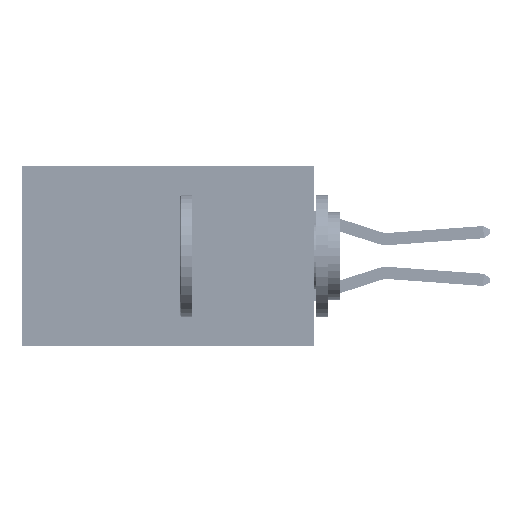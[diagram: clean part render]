
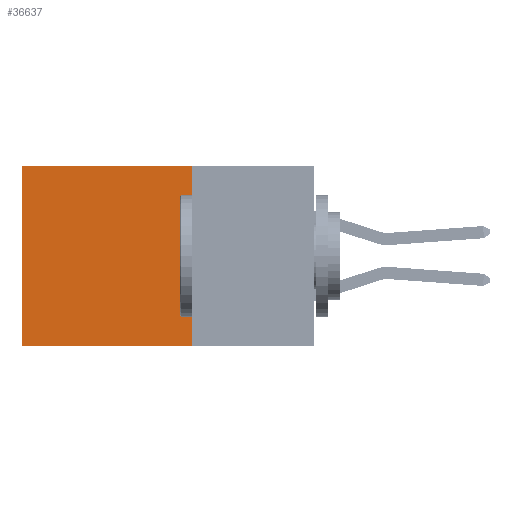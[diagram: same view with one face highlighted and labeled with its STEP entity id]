
A CAD part, left-side view. The second image highlights one B-rep face of the part: STEP entity #36637.
In plain terms, the highlighted planar face has unit normal (-1, 0, 0).
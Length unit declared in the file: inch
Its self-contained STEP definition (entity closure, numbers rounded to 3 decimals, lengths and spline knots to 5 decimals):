
#1279 = CARTESIAN_POINT ( 'NONE',  ( 0.2875, 0.25, 0. ) ) ;
#1438 = DIRECTION ( 'NONE',  ( 0., 1., 0. ) ) ;
#1686 = CARTESIAN_POINT ( 'NONE',  ( 0.2875, 0.6, 0. ) ) ;
#4145 = VERTEX_POINT ( 'NONE', #43274 ) ;
#5166 = DIRECTION ( 'NONE',  ( 1., 0., 0. ) ) ;
#6476 = CARTESIAN_POINT ( 'NONE',  ( 0.2875, 0.25, 0. ) ) ;
#7086 = LINE ( 'NONE', #35724, #45134 ) ;
#7599 = LINE ( 'NONE', #1686, #35656 ) ;
#8905 = ORIENTED_EDGE ( 'NONE', *, *, #9868, .T. ) ;
#8907 = PLANE ( 'NONE',  #10099 ) ;
#9868 = EDGE_CURVE ( 'NONE', #30553, #10388, #7599, .T. ) ;
#10099 = AXIS2_PLACEMENT_3D ( 'NONE', #1279, #5166, #31964 ) ;
#10341 = ORIENTED_EDGE ( 'NONE', *, *, #35509, .F. ) ;
#10388 = VERTEX_POINT ( 'NONE', #43488 ) ;
#11145 = VERTEX_POINT ( 'NONE', #36205 ) ;
#11567 = DIRECTION ( 'NONE',  ( 0., 1., 0. ) ) ;
#13233 = VECTOR ( 'NONE', #21738, 39.37008 ) ;
#17174 = DIRECTION ( 'NONE',  ( 0., 0., -1. ) ) ;
#19531 = ORIENTED_EDGE ( 'NONE', *, *, #38945, .T. ) ;
#21738 = DIRECTION ( 'NONE',  ( 0., 0., -1. ) ) ;
#23181 = VECTOR ( 'NONE', #11567, 39.37008 ) ;
#25744 = EDGE_LOOP ( 'NONE', ( #8905, #36055, #10341, #19531 ) ) ;
#30553 = VERTEX_POINT ( 'NONE', #30928 ) ;
#30922 = LINE ( 'NONE', #38148, #23181 ) ;
#30928 = CARTESIAN_POINT ( 'NONE',  ( 0.2875, 0.6, 0. ) ) ;
#31964 = DIRECTION ( 'NONE',  ( 0., 0., -1. ) ) ;
#35509 = EDGE_CURVE ( 'NONE', #4145, #11145, #42311, .T. ) ;
#35656 = VECTOR ( 'NONE', #17174, 39.37008 ) ;
#35724 = CARTESIAN_POINT ( 'NONE',  ( 0.2875, 0.25, 0. ) ) ;
#36055 = ORIENTED_EDGE ( 'NONE', *, *, #44611, .F. ) ;
#36205 = CARTESIAN_POINT ( 'NONE',  ( 0.2875, 0.25, -0.37 ) ) ;
#36637 = ADVANCED_FACE ( 'NONE', ( #41594 ), #8907, .F. ) ;
#38148 = CARTESIAN_POINT ( 'NONE',  ( 0.2875, 0.25, -0.37 ) ) ;
#38945 = EDGE_CURVE ( 'NONE', #4145, #30553, #7086, .T. ) ;
#41594 = FACE_OUTER_BOUND ( 'NONE', #25744, .T. ) ;
#42311 = LINE ( 'NONE', #6476, #13233 ) ;
#43274 = CARTESIAN_POINT ( 'NONE',  ( 0.2875, 0.25, 0. ) ) ;
#43488 = CARTESIAN_POINT ( 'NONE',  ( 0.2875, 0.6, -0.37 ) ) ;
#44611 = EDGE_CURVE ( 'NONE', #11145, #10388, #30922, .T. ) ;
#45134 = VECTOR ( 'NONE', #1438, 39.37008 ) ;
